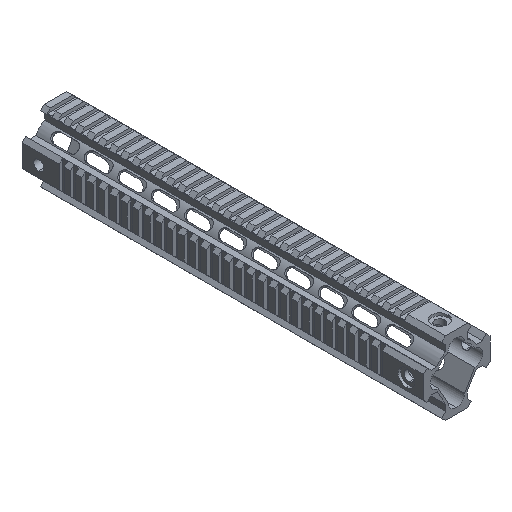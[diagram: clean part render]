
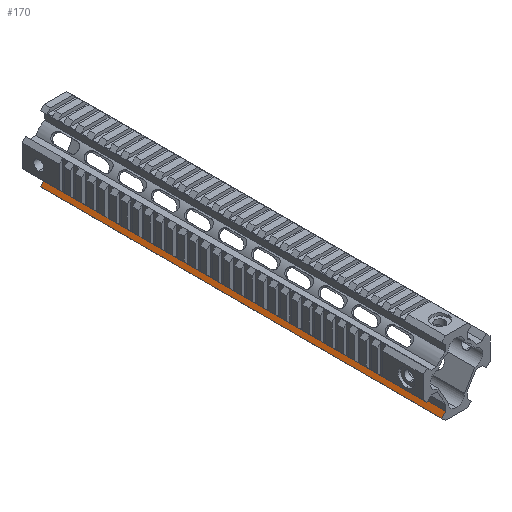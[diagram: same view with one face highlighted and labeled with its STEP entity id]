
A CAD part, isometric view. The second image highlights one B-rep face of the part: STEP entity #170.
In plain terms, the highlighted planar face has unit normal (-0.707, 0, 0.707).
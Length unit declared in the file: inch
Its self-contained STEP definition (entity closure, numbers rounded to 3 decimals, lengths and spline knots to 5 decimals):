
#170 = ADVANCED_FACE ( 'NONE', ( #17382 ), #25543, .F. ) ;
#465 = DIRECTION ( 'NONE',  ( 0.707, 0., -0.707 ) ) ;
#2870 = CARTESIAN_POINT ( 'NONE',  ( -0.44865, 12., -1.08135 ) ) ;
#4656 = VERTEX_POINT ( 'NONE', #20288 ) ;
#4739 = VERTEX_POINT ( 'NONE', #27792 ) ;
#6825 = ORIENTED_EDGE ( 'NONE', *, *, #34576, .F. ) ;
#10042 = EDGE_CURVE ( 'NONE', #4739, #4656, #37485, .T. ) ;
#11403 = VERTEX_POINT ( 'NONE', #14545 ) ;
#12973 = ORIENTED_EDGE ( 'NONE', *, *, #34219, .F. ) ;
#13364 = VECTOR ( 'NONE', #40074, 39.37008 ) ;
#13396 = VECTOR ( 'NONE', #25565, 39.37008 ) ;
#14545 = CARTESIAN_POINT ( 'NONE',  ( -0.44865, 12., -1.08135 ) ) ;
#15245 = LINE ( 'NONE', #33123, #30928 ) ;
#16857 = EDGE_CURVE ( 'NONE', #11403, #4739, #24915, .T. ) ;
#17382 = FACE_OUTER_BOUND ( 'NONE', #19976, .T. ) ;
#18101 = CARTESIAN_POINT ( 'NONE',  ( -0.32491, 12., -0.95761 ) ) ;
#19137 = ORIENTED_EDGE ( 'NONE', *, *, #10042, .T. ) ;
#19372 = CARTESIAN_POINT ( 'NONE',  ( -0.44865, 12., -1.08135 ) ) ;
#19976 = EDGE_LOOP ( 'NONE', ( #19137, #12973, #6825, #26913 ) ) ;
#20288 = CARTESIAN_POINT ( 'NONE',  ( -0.32491, 0., -0.95761 ) ) ;
#21732 = DIRECTION ( 'NONE',  ( 0., -1., 0. ) ) ;
#22525 = DIRECTION ( 'NONE',  ( -0.707, 0., -0.707 ) ) ;
#23597 = VERTEX_POINT ( 'NONE', #18101 ) ;
#24915 = LINE ( 'NONE', #2870, #33248 ) ;
#25543 = PLANE ( 'NONE',  #28136 ) ;
#25565 = DIRECTION ( 'NONE',  ( 0.707, 0., 0.707 ) ) ;
#26913 = ORIENTED_EDGE ( 'NONE', *, *, #16857, .T. ) ;
#27792 = CARTESIAN_POINT ( 'NONE',  ( -0.44865, 0., -1.08135 ) ) ;
#28136 = AXIS2_PLACEMENT_3D ( 'NONE', #19372, #465, #22525 ) ;
#30928 = VECTOR ( 'NONE', #36321, 39.37008 ) ;
#31476 = CARTESIAN_POINT ( 'NONE',  ( -0.44865, 0., -1.08135 ) ) ;
#33123 = CARTESIAN_POINT ( 'NONE',  ( -0.44865, 12., -1.08135 ) ) ;
#33248 = VECTOR ( 'NONE', #21732, 39.37008 ) ;
#34219 = EDGE_CURVE ( 'NONE', #23597, #4656, #37456, .T. ) ;
#34576 = EDGE_CURVE ( 'NONE', #11403, #23597, #15245, .T. ) ;
#36321 = DIRECTION ( 'NONE',  ( 0.707, 0., 0.707 ) ) ;
#37456 = LINE ( 'NONE', #40211, #13364 ) ;
#37485 = LINE ( 'NONE', #31476, #13396 ) ;
#40074 = DIRECTION ( 'NONE',  ( 0., -1., 0. ) ) ;
#40211 = CARTESIAN_POINT ( 'NONE',  ( -0.32491, 12., -0.95761 ) ) ;
